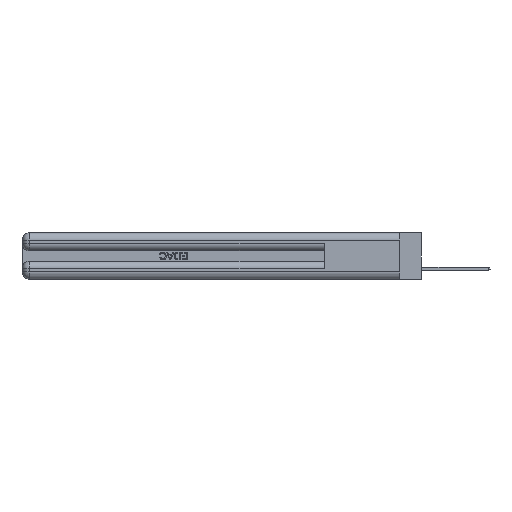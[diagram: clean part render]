
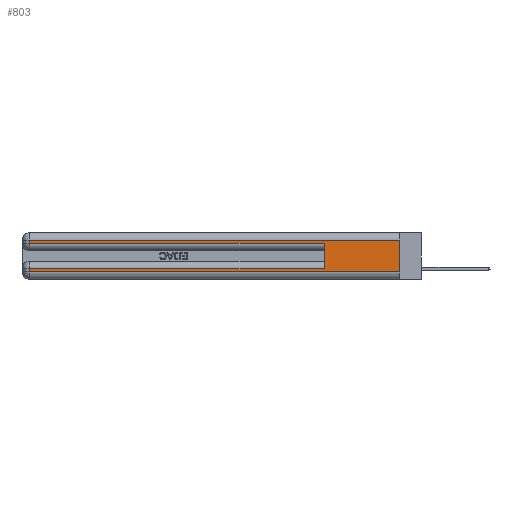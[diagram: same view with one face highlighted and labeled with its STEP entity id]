
A CAD part, left-side view. The second image highlights one B-rep face of the part: STEP entity #803.
In plain terms, the highlighted planar face has unit normal (-1, 0, 0).
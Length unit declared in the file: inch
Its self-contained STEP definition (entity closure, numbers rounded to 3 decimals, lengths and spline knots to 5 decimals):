
#207 = CARTESIAN_POINT ( 'NONE',  ( 0., 0.6, 0.145 ) ) ;
#336 = VERTEX_POINT ( 'NONE', #17626 ) ;
#803 = ADVANCED_FACE ( 'NONE', ( #19639 ), #7435, .F. ) ;
#1204 = VECTOR ( 'NONE', #3834, 39.37008 ) ;
#1500 = DIRECTION ( 'NONE',  ( 1., 0., 0. ) ) ;
#2329 = CARTESIAN_POINT ( 'NONE',  ( 0., 0., 0.085 ) ) ;
#2575 = VERTEX_POINT ( 'NONE', #43798 ) ;
#2684 = LINE ( 'NONE', #39220, #43414 ) ;
#2701 = CARTESIAN_POINT ( 'NONE',  ( 0., 0., 0.37 ) ) ;
#3774 = VECTOR ( 'NONE', #12893, 39.37008 ) ;
#3834 = DIRECTION ( 'NONE',  ( 0., -1., 0. ) ) ;
#3984 = EDGE_CURVE ( 'NONE', #336, #17121, #38536, .T. ) ;
#4395 = LINE ( 'NONE', #25424, #21486 ) ;
#4997 = DIRECTION ( 'NONE',  ( 0., 0., -1. ) ) ;
#5521 = VECTOR ( 'NONE', #20494, 39.37008 ) ;
#6417 = DIRECTION ( 'NONE',  ( 0., 0., -1. ) ) ;
#6570 = LINE ( 'NONE', #207, #5521 ) ;
#6795 = CARTESIAN_POINT ( 'NONE',  ( 0., 0.6, 0.285 ) ) ;
#7181 = DIRECTION ( 'NONE',  ( 0., 1., 0. ) ) ;
#7435 = PLANE ( 'NONE',  #28237 ) ;
#10754 = ORIENTED_EDGE ( 'NONE', *, *, #13184, .T. ) ;
#12449 = LINE ( 'NONE', #20696, #1204 ) ;
#12893 = DIRECTION ( 'NONE',  ( 0., 1., 0. ) ) ;
#13028 = ORIENTED_EDGE ( 'NONE', *, *, #37884, .T. ) ;
#13184 = EDGE_CURVE ( 'NONE', #17121, #2575, #4395, .T. ) ;
#13924 = LINE ( 'NONE', #2329, #3774 ) ;
#14593 = DIRECTION ( 'NONE',  ( 0., 0., -1. ) ) ;
#15921 = ORIENTED_EDGE ( 'NONE', *, *, #16836, .T. ) ;
#16538 = ORIENTED_EDGE ( 'NONE', *, *, #30881, .F. ) ;
#16836 = EDGE_CURVE ( 'NONE', #2575, #27523, #2684, .T. ) ;
#17121 = VERTEX_POINT ( 'NONE', #39770 ) ;
#17626 = CARTESIAN_POINT ( 'NONE',  ( 0., 0., 0.31 ) ) ;
#17927 = EDGE_LOOP ( 'NONE', ( #40479, #29262, #10754, #15921, #16538, #13028, #40759, #44286 ) ) ;
#18004 = VERTEX_POINT ( 'NONE', #43193 ) ;
#19639 = FACE_OUTER_BOUND ( 'NONE', #17927, .T. ) ;
#20135 = VERTEX_POINT ( 'NONE', #40599 ) ;
#20347 = VECTOR ( 'NONE', #7181, 39.37008 ) ;
#20494 = DIRECTION ( 'NONE',  ( 0., 0., 1. ) ) ;
#20696 = CARTESIAN_POINT ( 'NONE',  ( 0., 0., 0.06 ) ) ;
#21486 = VECTOR ( 'NONE', #4997, 39.37008 ) ;
#22050 = CARTESIAN_POINT ( 'NONE',  ( 0., 0., 0.06 ) ) ;
#23420 = DIRECTION ( 'NONE',  ( 0., 0., -1. ) ) ;
#24443 = EDGE_CURVE ( 'NONE', #336, #40098, #37661, .T. ) ;
#24896 = VERTEX_POINT ( 'NONE', #42932 ) ;
#25424 = CARTESIAN_POINT ( 'NONE',  ( 0., 2.94, 0.37 ) ) ;
#25858 = LINE ( 'NONE', #37384, #30184 ) ;
#27523 = VERTEX_POINT ( 'NONE', #6795 ) ;
#28237 = AXIS2_PLACEMENT_3D ( 'NONE', #35076, #1500, #14593 ) ;
#29015 = DIRECTION ( 'NONE',  ( 0., -1., 0. ) ) ;
#29262 = ORIENTED_EDGE ( 'NONE', *, *, #3984, .T. ) ;
#30184 = VECTOR ( 'NONE', #6417, 39.37008 ) ;
#30881 = EDGE_CURVE ( 'NONE', #18004, #27523, #6570, .T. ) ;
#31486 = CARTESIAN_POINT ( 'NONE',  ( 0., 0., 0.31 ) ) ;
#35076 = CARTESIAN_POINT ( 'NONE',  ( 0., 0., 0.37 ) ) ;
#36061 = VECTOR ( 'NONE', #23420, 39.37008 ) ;
#36079 = EDGE_CURVE ( 'NONE', #24896, #20135, #25858, .T. ) ;
#36854 = EDGE_CURVE ( 'NONE', #20135, #40098, #12449, .T. ) ;
#37384 = CARTESIAN_POINT ( 'NONE',  ( 0., 2.94, 0.37 ) ) ;
#37661 = LINE ( 'NONE', #2701, #36061 ) ;
#37884 = EDGE_CURVE ( 'NONE', #18004, #24896, #13924, .T. ) ;
#38536 = LINE ( 'NONE', #31486, #20347 ) ;
#39220 = CARTESIAN_POINT ( 'NONE',  ( 0., 0., 0.285 ) ) ;
#39770 = CARTESIAN_POINT ( 'NONE',  ( 0., 2.94, 0.31 ) ) ;
#40098 = VERTEX_POINT ( 'NONE', #22050 ) ;
#40479 = ORIENTED_EDGE ( 'NONE', *, *, #24443, .F. ) ;
#40599 = CARTESIAN_POINT ( 'NONE',  ( 0., 2.94, 0.06 ) ) ;
#40759 = ORIENTED_EDGE ( 'NONE', *, *, #36079, .T. ) ;
#42932 = CARTESIAN_POINT ( 'NONE',  ( 0., 2.94, 0.085 ) ) ;
#43193 = CARTESIAN_POINT ( 'NONE',  ( 0., 0.6, 0.085 ) ) ;
#43414 = VECTOR ( 'NONE', #29015, 39.37008 ) ;
#43798 = CARTESIAN_POINT ( 'NONE',  ( 0., 2.94, 0.285 ) ) ;
#44286 = ORIENTED_EDGE ( 'NONE', *, *, #36854, .T. ) ;
